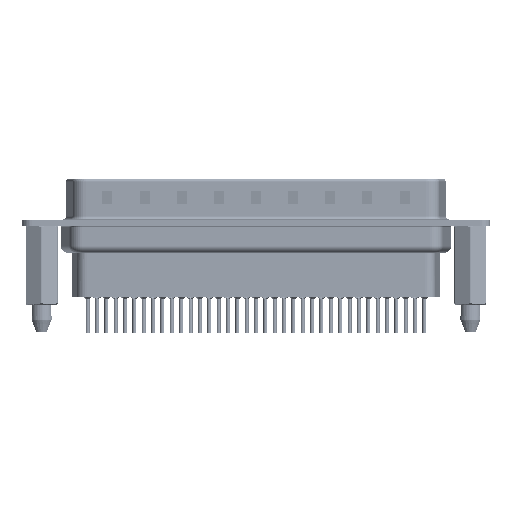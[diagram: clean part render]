
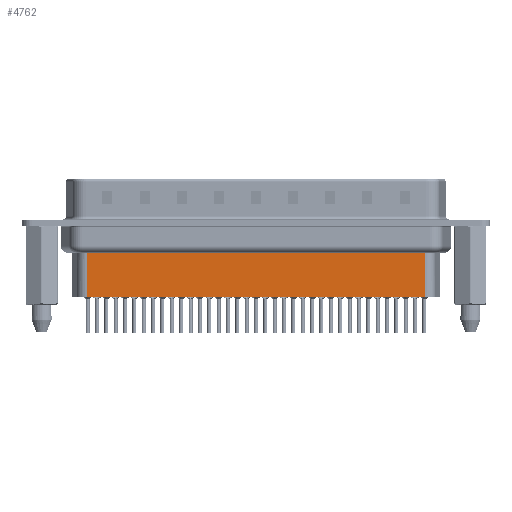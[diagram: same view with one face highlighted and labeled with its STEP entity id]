
A CAD part, front view. The second image highlights one B-rep face of the part: STEP entity #4762.
In plain terms, the highlighted planar face has unit normal (0, -1, 0).
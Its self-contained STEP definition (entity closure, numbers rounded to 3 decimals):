
#404 = LINE ( 'NONE', #20101, #23258 ) ;
#2111 = CARTESIAN_POINT ( 'NONE',  ( 56.794, -3.5, -4.097 ) ) ;
#2398 = VERTEX_POINT ( 'NONE', #2111 ) ;
#2858 = ORIENTED_EDGE ( 'NONE', *, *, #8066, .T. ) ;
#3547 = EDGE_CURVE ( 'NONE', #2398, #7970, #28398, .T. ) ;
#4075 = VECTOR ( 'NONE', #15533, 1000. ) ;
#4762 = ADVANCED_FACE ( 'NONE', ( #30505 ), #25460, .T. ) ;
#5277 = CARTESIAN_POINT ( 'NONE',  ( 6.706, -3.5, -3.1 ) ) ;
#6681 = EDGE_CURVE ( 'NONE', #28958, #11370, #404, .T. ) ;
#7970 = VERTEX_POINT ( 'NONE', #14170 ) ;
#8066 = EDGE_CURVE ( 'NONE', #7970, #11370, #26690, .T. ) ;
#8193 = DIRECTION ( 'NONE',  ( 1., 0., 0. ) ) ;
#9763 = ORIENTED_EDGE ( 'NONE', *, *, #6681, .F. ) ;
#11370 = VERTEX_POINT ( 'NONE', #29736 ) ;
#12271 = ORIENTED_EDGE ( 'NONE', *, *, #3547, .T. ) ;
#12355 = VECTOR ( 'NONE', #29131, 1000. ) ;
#12824 = LINE ( 'NONE', #20136, #21421 ) ;
#13806 = AXIS2_PLACEMENT_3D ( 'NONE', #5277, #30667, #8193 ) ;
#13858 = EDGE_CURVE ( 'NONE', #2398, #28958, #12824, .T. ) ;
#14170 = CARTESIAN_POINT ( 'NONE',  ( 6.706, -3.5, -4.097 ) ) ;
#15533 = DIRECTION ( 'NONE',  ( -1., 0., 0. ) ) ;
#19268 = ORIENTED_EDGE ( 'NONE', *, *, #13858, .F. ) ;
#20101 = CARTESIAN_POINT ( 'NONE',  ( 6.706, -3.5, -10.95 ) ) ;
#20136 = CARTESIAN_POINT ( 'NONE',  ( 56.794, -3.5, -3.1 ) ) ;
#20525 = EDGE_LOOP ( 'NONE', ( #19268, #12271, #2858, #9763 ) ) ;
#21421 = VECTOR ( 'NONE', #28122, 1000. ) ;
#23194 = CARTESIAN_POINT ( 'NONE',  ( 6.459, -3.5, -4.097 ) ) ;
#23258 = VECTOR ( 'NONE', #29868, 1000. ) ;
#25460 = PLANE ( 'NONE',  #13806 ) ;
#26690 = LINE ( 'NONE', #28816, #12355 ) ;
#28122 = DIRECTION ( 'NONE',  ( 0., 0., -1. ) ) ;
#28398 = LINE ( 'NONE', #23194, #4075 ) ;
#28407 = CARTESIAN_POINT ( 'NONE',  ( 56.794, -3.5, -10.95 ) ) ;
#28816 = CARTESIAN_POINT ( 'NONE',  ( 6.706, -3.5, -3.1 ) ) ;
#28958 = VERTEX_POINT ( 'NONE', #28407 ) ;
#29131 = DIRECTION ( 'NONE',  ( 0., 0., -1. ) ) ;
#29736 = CARTESIAN_POINT ( 'NONE',  ( 6.706, -3.5, -10.95 ) ) ;
#29868 = DIRECTION ( 'NONE',  ( -1., 0., 0. ) ) ;
#30505 = FACE_OUTER_BOUND ( 'NONE', #20525, .T. ) ;
#30667 = DIRECTION ( 'NONE',  ( 0., -1., 0. ) ) ;
